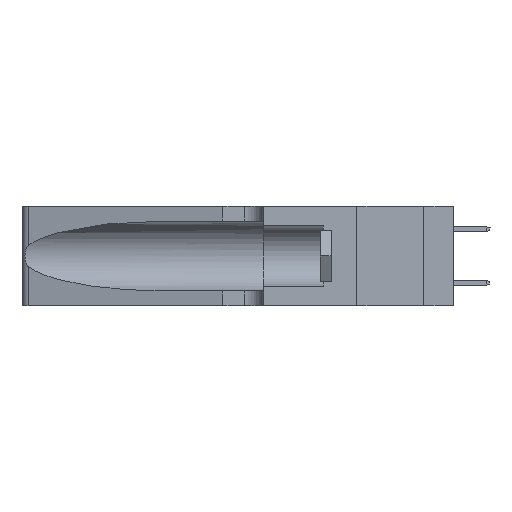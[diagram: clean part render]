
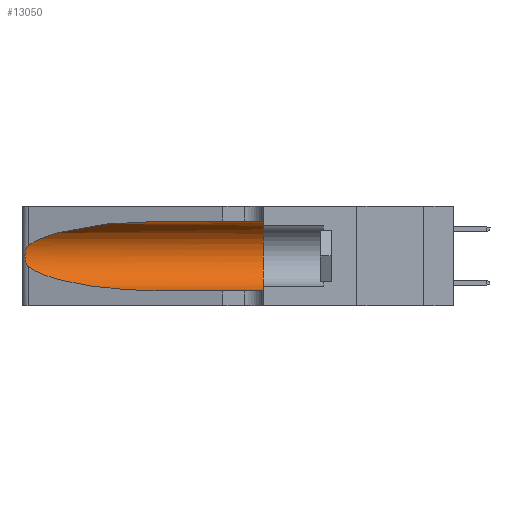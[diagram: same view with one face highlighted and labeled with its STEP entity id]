
A CAD part, left-side view. The second image highlights one B-rep face of the part: STEP entity #13050.
In plain terms, the highlighted cylindrical face has radius 3.308 mm (diameter 6.617 mm), a partial arc.
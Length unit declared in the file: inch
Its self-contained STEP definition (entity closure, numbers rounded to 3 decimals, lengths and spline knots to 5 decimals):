
#332 = VERTEX_POINT ( 'NONE', #14080 ) ;
#630 = CARTESIAN_POINT ( 'NONE',  ( 0.1305, 0.72297, 0.31525 ) ) ;
#859 = DIRECTION ( 'NONE',  ( 0., 1., 0. ) ) ;
#867 = CARTESIAN_POINT ( 'NONE',  ( 0.26017, 1.23833, 0.17102 ) ) ;
#1004 = CARTESIAN_POINT ( 'NONE',  ( 0.1305, 0.35, 0.05475 ) ) ;
#2422 = AXIS2_PLACEMENT_3D ( 'NONE', #16648, #859, #6859 ) ;
#2642 = DIRECTION ( 'NONE',  ( 0., -1., 0. ) ) ;
#2652 = CARTESIAN_POINT ( 'NONE',  ( 0.18966, 0.96281, 0.05475 ) ) ;
#3307 = ORIENTED_EDGE ( 'NONE', *, *, #8933, .T. ) ;
#3428 = AXIS2_PLACEMENT_3D ( 'NONE', #10674, #4584, #10781 ) ;
#4168 = CARTESIAN_POINT ( 'NONE',  ( 0.25487, 1.22718, 0.22369 ) ) ;
#4584 = DIRECTION ( 'NONE',  ( 0., -1., 0. ) ) ;
#4906 = DIRECTION ( 'NONE',  ( 0., -1., 0. ) ) ;
#5145 = CARTESIAN_POINT ( 'NONE',  ( 0.25487, 1.22718, 0.22369 ) ) ;
#5425 = CARTESIAN_POINT ( 'NONE',  ( 0.25854, 1.2359, 0.20912 ) ) ;
#5512 = CARTESIAN_POINT ( 'NONE',  ( 0.26075, 1.23896, 0.19203 ) ) ;
#6354 = CIRCLE ( 'NONE', #2422, 0.13025 ) ;
#6464 = LINE ( 'NONE', #12770, #16338 ) ;
#6499 = VERTEX_POINT ( 'NONE', #11602 ) ;
#6853 = VERTEX_POINT ( 'NONE', #630 ) ;
#6859 = DIRECTION ( 'NONE',  ( 0., 0., 1. ) ) ;
#7277 = CARTESIAN_POINT ( 'NONE',  ( 0.25555, 1.22993, 0.14849 ) ) ;
#7735 = VECTOR ( 'NONE', #2642, 39.37008 ) ;
#7790 = ORIENTED_EDGE ( 'NONE', *, *, #12209, .F. ) ;
#8481 = VERTEX_POINT ( 'NONE', #5145 ) ;
#8732 = CARTESIAN_POINT ( 'NONE',  ( 0.26018, 1.23835, 0.19895 ) ) ;
#8834 = CARTESIAN_POINT ( 'NONE',  ( 0.26075, 1.23896, 0.178 ) ) ;
#8927 = CARTESIAN_POINT ( 'NONE',  ( 0.25639, 1.23186, 0.15144 ) ) ;
#8933 = EDGE_CURVE ( 'NONE', #8481, #19528, #17593, .T. ) ;
#9421 = ORIENTED_EDGE ( 'NONE', *, *, #17017, .T. ) ;
#9551 = FACE_OUTER_BOUND ( 'NONE', #13829, .T. ) ;
#9731 = CARTESIAN_POINT ( 'NONE',  ( 0.25487, 1.22718, 0.22369 ) ) ;
#10211 = EDGE_CURVE ( 'NONE', #6853, #8481, #15329, .T. ) ;
#10261 = CARTESIAN_POINT ( 'NONE',  ( 0.25787, 1.23484, 0.2124 ) ) ;
#10277 = CARTESIAN_POINT ( 'NONE',  ( 0.25487, 1.22718, 0.14631 ) ) ;
#10355 = CARTESIAN_POINT ( 'NONE',  ( 0.25789, 1.23486, 0.15765 ) ) ;
#10577 = CARTESIAN_POINT ( 'NONE',  ( 0.2373, 1.15595, 0.08982 ) ) ;
#10674 = CARTESIAN_POINT ( 'NONE',  ( 0.1305, 1.61858, 0.185 ) ) ;
#10781 = DIRECTION ( 'NONE',  ( 0., 0., -1. ) ) ;
#11099 = CYLINDRICAL_SURFACE ( 'NONE', #3428, 0.13025 ) ;
#11602 = CARTESIAN_POINT ( 'NONE',  ( 0.1305, 0.72297, 0.05475 ) ) ;
#12143 = CARTESIAN_POINT ( 'NONE',  ( 0.1305, 0.72297, 0.05475 ) ) ;
#12162 = CARTESIAN_POINT ( 'NONE',  ( 0.25487, 1.22718, 0.14631 ) ) ;
#12209 = EDGE_CURVE ( 'NONE', #332, #19630, #6354, .T. ) ;
#12356 = ORIENTED_EDGE ( 'NONE', *, *, #10211, .T. ) ;
#12770 = CARTESIAN_POINT ( 'NONE',  ( 0.1305, 1.61858, 0.05475 ) ) ;
#13050 = ADVANCED_FACE ( 'NONE', ( #9551 ), #11099, .F. ) ;
#13181 = CARTESIAN_POINT ( 'NONE',  ( 0.25856, 1.23593, 0.16098 ) ) ;
#13339 =( BOUNDED_CURVE ( )  B_SPLINE_CURVE ( 3, ( #10277, #10577, #2652, #12143 ),
 .UNSPECIFIED., .F., .T. ) 
 B_SPLINE_CURVE_WITH_KNOTS ( ( 4, 4 ),
 ( 3.44316, 4.71239 ),
 .UNSPECIFIED. ) 
 CURVE ( )  GEOMETRIC_REPRESENTATION_ITEM ( )  RATIONAL_B_SPLINE_CURVE ( ( 1., 0.87, 0.87, 1. ) ) 
 REPRESENTATION_ITEM ( '' )  );
#13368 = CARTESIAN_POINT ( 'NONE',  ( 0.25639, 1.23184, 0.21858 ) ) ;
#13552 = ORIENTED_EDGE ( 'NONE', *, *, #14868, .T. ) ;
#13829 = EDGE_LOOP ( 'NONE', ( #12356, #3307, #13552, #9421, #7790, #19041 ) ) ;
#14080 = CARTESIAN_POINT ( 'NONE',  ( 0.1305, 0.35, 0.31525 ) ) ;
#14166 = EDGE_CURVE ( 'NONE', #6853, #332, #19761, .T. ) ;
#14603 = CARTESIAN_POINT ( 'NONE',  ( 0.18966, 0.96281, 0.31525 ) ) ;
#14806 = CARTESIAN_POINT ( 'NONE',  ( 0.1305, 0.72297, 0.31525 ) ) ;
#14868 = EDGE_CURVE ( 'NONE', #19528, #6499, #13339, .T. ) ;
#15329 =( BOUNDED_CURVE ( )  B_SPLINE_CURVE ( 3, ( #14806, #14603, #19225, #9731 ),
 .UNSPECIFIED., .F., .T. ) 
 B_SPLINE_CURVE_WITH_KNOTS ( ( 4, 4 ),
 ( 1.5708, 2.84003 ),
 .UNSPECIFIED. ) 
 CURVE ( )  GEOMETRIC_REPRESENTATION_ITEM ( )  RATIONAL_B_SPLINE_CURVE ( ( 1., 0.87, 0.87, 1. ) ) 
 REPRESENTATION_ITEM ( '' )  );
#16338 = VECTOR ( 'NONE', #4906, 39.37008 ) ;
#16648 = CARTESIAN_POINT ( 'NONE',  ( 0.1305, 0.35, 0.185 ) ) ;
#16750 = CARTESIAN_POINT ( 'NONE',  ( 0.25555, 1.22994, 0.2215 ) ) ;
#17017 = EDGE_CURVE ( 'NONE', #6499, #19630, #6464, .T. ) ;
#17593 = B_SPLINE_CURVE_WITH_KNOTS ( 'NONE', 3,
 ( #4168, #16750, #13368, #10261, #5425, #8732, #5512, #8834, #867, #13181, #10355, #8927, #7277, #19643 ),
 .UNSPECIFIED., .F., .F.,
 ( 4, 2, 2, 2, 2, 2, 4 ),
 ( 0., 0.00027, 0.00053, 0.00107, 0.0016, 0.00187, 0.00214 ),
 .UNSPECIFIED. ) ;
#18240 = CARTESIAN_POINT ( 'NONE',  ( 0.1305, 1.61858, 0.31525 ) ) ;
#19041 = ORIENTED_EDGE ( 'NONE', *, *, #14166, .F. ) ;
#19225 = CARTESIAN_POINT ( 'NONE',  ( 0.2373, 1.15595, 0.28018 ) ) ;
#19528 = VERTEX_POINT ( 'NONE', #12162 ) ;
#19630 = VERTEX_POINT ( 'NONE', #1004 ) ;
#19643 = CARTESIAN_POINT ( 'NONE',  ( 0.25487, 1.22718, 0.14631 ) ) ;
#19761 = LINE ( 'NONE', #18240, #7735 ) ;
